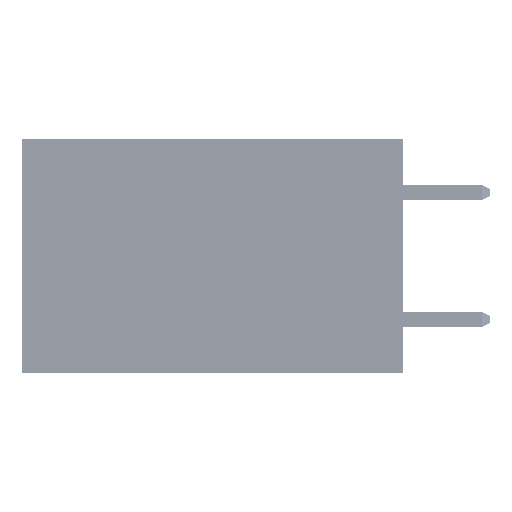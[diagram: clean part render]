
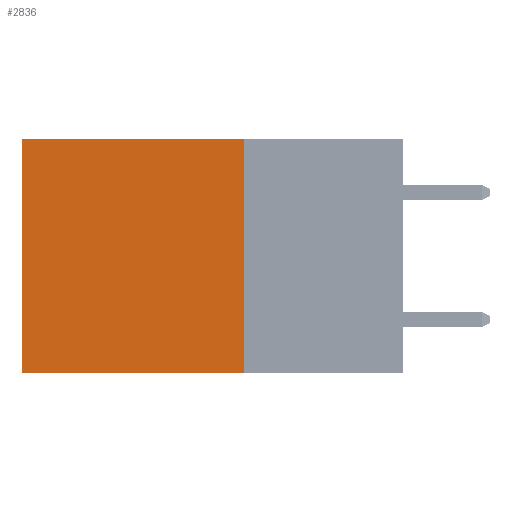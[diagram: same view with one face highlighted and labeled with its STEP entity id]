
A CAD part, left-side view. The second image highlights one B-rep face of the part: STEP entity #2836.
In plain terms, the highlighted planar face has unit normal (-1, 0, 0).
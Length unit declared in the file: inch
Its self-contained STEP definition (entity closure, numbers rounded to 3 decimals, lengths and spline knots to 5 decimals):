
#910 = LINE ( 'NONE', #4637, #50815 ) ;
#983 = CARTESIAN_POINT ( 'NONE',  ( 0.2875, 0.25, 0. ) ) ;
#1136 = CARTESIAN_POINT ( 'NONE',  ( 0.2875, 0.6, -0.37 ) ) ;
#1509 = FACE_OUTER_BOUND ( 'NONE', #17454, .T. ) ;
#2836 = ADVANCED_FACE ( 'NONE', ( #1509 ), #8938, .F. ) ;
#4637 = CARTESIAN_POINT ( 'NONE',  ( 0.2875, 0.25, 0. ) ) ;
#6569 = EDGE_CURVE ( 'NONE', #7731, #36055, #19330, .T. ) ;
#7731 = VERTEX_POINT ( 'NONE', #39723 ) ;
#8005 = CARTESIAN_POINT ( 'NONE',  ( 0.2875, 0.6, 0. ) ) ;
#8938 = PLANE ( 'NONE',  #25535 ) ;
#9322 = DIRECTION ( 'NONE',  ( 0., 0., -1. ) ) ;
#11290 = LINE ( 'NONE', #27977, #44234 ) ;
#16738 = DIRECTION ( 'NONE',  ( 0., 1., 0. ) ) ;
#17454 = EDGE_LOOP ( 'NONE', ( #30156, #40023, #49500, #23639 ) ) ;
#17485 = VERTEX_POINT ( 'NONE', #40590 ) ;
#19330 = LINE ( 'NONE', #31794, #33350 ) ;
#19602 = DIRECTION ( 'NONE',  ( 0., 1., 0. ) ) ;
#21507 = CARTESIAN_POINT ( 'NONE',  ( 0.2875, 0.6, 0. ) ) ;
#22782 = EDGE_CURVE ( 'NONE', #17485, #29708, #11290, .T. ) ;
#23639 = ORIENTED_EDGE ( 'NONE', *, *, #6569, .T. ) ;
#25352 = DIRECTION ( 'NONE',  ( 1., 0., 0. ) ) ;
#25535 = AXIS2_PLACEMENT_3D ( 'NONE', #983, #25352, #41501 ) ;
#27977 = CARTESIAN_POINT ( 'NONE',  ( 0.2875, 0.25, -0.37 ) ) ;
#29708 = VERTEX_POINT ( 'NONE', #1136 ) ;
#30156 = ORIENTED_EDGE ( 'NONE', *, *, #43108, .T. ) ;
#31794 = CARTESIAN_POINT ( 'NONE',  ( 0.2875, 0.25, 0. ) ) ;
#33350 = VECTOR ( 'NONE', #19602, 39.37008 ) ;
#36055 = VERTEX_POINT ( 'NONE', #8005 ) ;
#37669 = LINE ( 'NONE', #21507, #39751 ) ;
#39723 = CARTESIAN_POINT ( 'NONE',  ( 0.2875, 0.25, 0. ) ) ;
#39751 = VECTOR ( 'NONE', #9322, 39.37008 ) ;
#40023 = ORIENTED_EDGE ( 'NONE', *, *, #22782, .F. ) ;
#40590 = CARTESIAN_POINT ( 'NONE',  ( 0.2875, 0.25, -0.37 ) ) ;
#41501 = DIRECTION ( 'NONE',  ( 0., 0., -1. ) ) ;
#41697 = DIRECTION ( 'NONE',  ( 0., 0., -1. ) ) ;
#43108 = EDGE_CURVE ( 'NONE', #36055, #29708, #37669, .T. ) ;
#44234 = VECTOR ( 'NONE', #16738, 39.37008 ) ;
#46411 = EDGE_CURVE ( 'NONE', #7731, #17485, #910, .T. ) ;
#49500 = ORIENTED_EDGE ( 'NONE', *, *, #46411, .F. ) ;
#50815 = VECTOR ( 'NONE', #41697, 39.37008 ) ;
